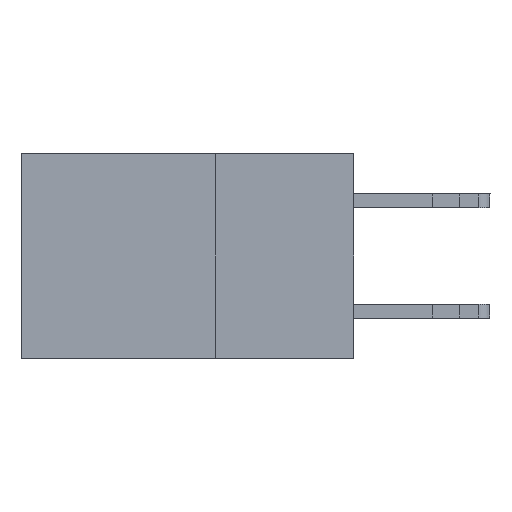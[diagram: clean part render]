
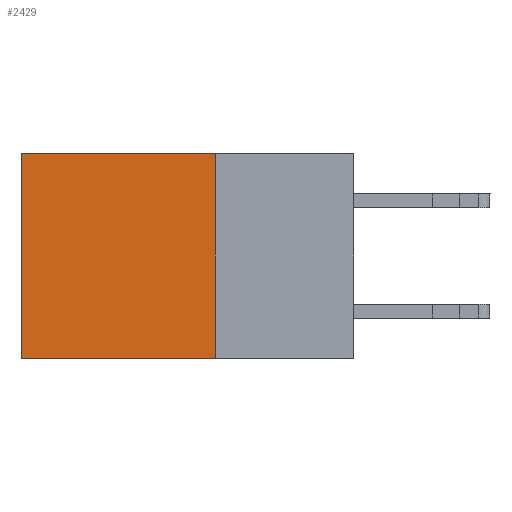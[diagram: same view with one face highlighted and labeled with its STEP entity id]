
A CAD part, left-side view. The second image highlights one B-rep face of the part: STEP entity #2429.
In plain terms, the highlighted planar face has unit normal (-1, 0, 0).
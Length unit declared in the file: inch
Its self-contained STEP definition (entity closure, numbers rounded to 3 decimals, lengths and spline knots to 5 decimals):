
#16 = CARTESIAN_POINT ( 'NONE',  ( 0.2875, 0.25, 0. ) ) ;
#597 = VERTEX_POINT ( 'NONE', #7327 ) ;
#730 = CARTESIAN_POINT ( 'NONE',  ( 0.2875, 0.25, 0. ) ) ;
#818 = VERTEX_POINT ( 'NONE', #4206 ) ;
#836 = EDGE_CURVE ( 'NONE', #818, #13853, #14907, .T. ) ;
#1584 = CARTESIAN_POINT ( 'NONE',  ( 0.2875, 0.6, -0.37 ) ) ;
#1863 = DIRECTION ( 'NONE',  ( 0., 0., -1. ) ) ;
#2429 = ADVANCED_FACE ( 'NONE', ( #12868 ), #15071, .F. ) ;
#2739 = LINE ( 'NONE', #730, #16635 ) ;
#2748 = DIRECTION ( 'NONE',  ( 0., 1., 0. ) ) ;
#3903 = DIRECTION ( 'NONE',  ( 1., 0., 0. ) ) ;
#3911 = ORIENTED_EDGE ( 'NONE', *, *, #6421, .F. ) ;
#3971 = EDGE_LOOP ( 'NONE', ( #16461, #6944, #3911, #12190 ) ) ;
#4206 = CARTESIAN_POINT ( 'NONE',  ( 0.2875, 0.25, 0. ) ) ;
#4298 = CARTESIAN_POINT ( 'NONE',  ( 0.2875, 0.6, 0. ) ) ;
#5299 = DIRECTION ( 'NONE',  ( 0., 0., -1. ) ) ;
#6421 = EDGE_CURVE ( 'NONE', #818, #597, #2739, .T. ) ;
#6944 = ORIENTED_EDGE ( 'NONE', *, *, #13789, .F. ) ;
#7046 = DIRECTION ( 'NONE',  ( 0., 1., 0. ) ) ;
#7327 = CARTESIAN_POINT ( 'NONE',  ( 0.2875, 0.25, -0.37 ) ) ;
#7378 = AXIS2_PLACEMENT_3D ( 'NONE', #16, #3903, #5299 ) ;
#9222 = LINE ( 'NONE', #12312, #13287 ) ;
#10171 = VECTOR ( 'NONE', #7046, 39.37008 ) ;
#10466 = DIRECTION ( 'NONE',  ( 0., 0., -1. ) ) ;
#12161 = VECTOR ( 'NONE', #1863, 39.37008 ) ;
#12190 = ORIENTED_EDGE ( 'NONE', *, *, #836, .T. ) ;
#12312 = CARTESIAN_POINT ( 'NONE',  ( 0.2875, 0.25, -0.37 ) ) ;
#12868 = FACE_OUTER_BOUND ( 'NONE', #3971, .T. ) ;
#13287 = VECTOR ( 'NONE', #2748, 39.37008 ) ;
#13789 = EDGE_CURVE ( 'NONE', #597, #16919, #9222, .T. ) ;
#13853 = VERTEX_POINT ( 'NONE', #4298 ) ;
#14907 = LINE ( 'NONE', #15251, #10171 ) ;
#15071 = PLANE ( 'NONE',  #7378 ) ;
#15251 = CARTESIAN_POINT ( 'NONE',  ( 0.2875, 0.25, 0. ) ) ;
#15776 = EDGE_CURVE ( 'NONE', #13853, #16919, #16259, .T. ) ;
#16259 = LINE ( 'NONE', #17031, #12161 ) ;
#16461 = ORIENTED_EDGE ( 'NONE', *, *, #15776, .T. ) ;
#16635 = VECTOR ( 'NONE', #10466, 39.37008 ) ;
#16919 = VERTEX_POINT ( 'NONE', #1584 ) ;
#17031 = CARTESIAN_POINT ( 'NONE',  ( 0.2875, 0.6, 0. ) ) ;
